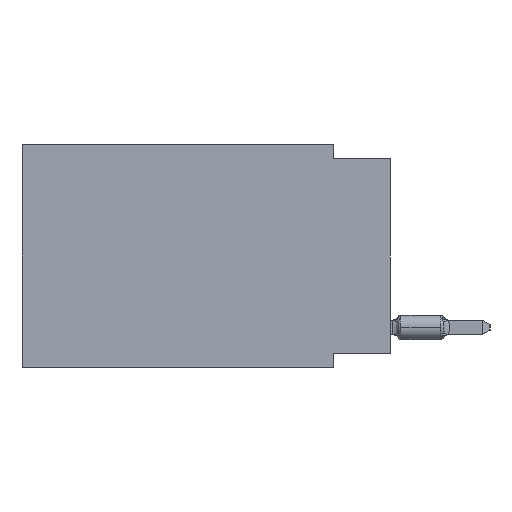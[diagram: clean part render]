
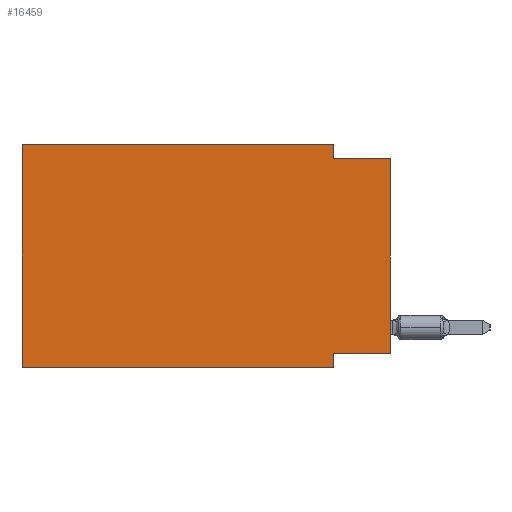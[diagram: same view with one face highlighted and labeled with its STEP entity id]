
A CAD part, left-side view. The second image highlights one B-rep face of the part: STEP entity #16459.
In plain terms, the highlighted planar face has unit normal (-1, 0, 0).
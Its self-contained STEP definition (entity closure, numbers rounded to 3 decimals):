
#486 = EDGE_CURVE ( 'NONE', #56220, #3566, #26985, .T. ) ;
#1985 = CARTESIAN_POINT ( 'NONE',  ( 0., 0., 0. ) ) ;
#2915 = ORIENTED_EDGE ( 'NONE', *, *, #71322, .F. ) ;
#3430 = PLANE ( 'NONE',  #68367 ) ;
#3566 = VERTEX_POINT ( 'NONE', #26659 ) ;
#4376 = VECTOR ( 'NONE', #16725, 1000. ) ;
#4615 = VERTEX_POINT ( 'NONE', #43589 ) ;
#5966 = CARTESIAN_POINT ( 'NONE',  ( 0., 0., -0.635 ) ) ;
#5991 = VERTEX_POINT ( 'NONE', #57848 ) ;
#6967 = VECTOR ( 'NONE', #25536, 1000. ) ;
#7829 = LINE ( 'NONE', #36813, #31061 ) ;
#8738 = CARTESIAN_POINT ( 'NONE',  ( 0., 2.54, -0.635 ) ) ;
#9152 = LINE ( 'NONE', #67476, #35748 ) ;
#10105 = VECTOR ( 'NONE', #44324, 1000. ) ;
#14427 = CARTESIAN_POINT ( 'NONE',  ( 0., 2.54, -9.906 ) ) ;
#15564 = EDGE_CURVE ( 'NONE', #56220, #51769, #19150, .T. ) ;
#15979 = LINE ( 'NONE', #45315, #4376 ) ;
#16459 = ADVANCED_FACE ( 'NONE', ( #54260 ), #3430, .F. ) ;
#16725 = DIRECTION ( 'NONE',  ( 0., -1., 0. ) ) ;
#19124 = DIRECTION ( 'NONE',  ( 0., 0., -1. ) ) ;
#19150 = LINE ( 'NONE', #37577, #6967 ) ;
#19627 = EDGE_CURVE ( 'NONE', #5991, #39199, #70482, .T. ) ;
#21343 = CARTESIAN_POINT ( 'NONE',  ( 0., 0., -0.635 ) ) ;
#25536 = DIRECTION ( 'NONE',  ( 0., -1., 0. ) ) ;
#25578 = VECTOR ( 'NONE', #36987, 1000. ) ;
#26659 = CARTESIAN_POINT ( 'NONE',  ( 0., 16.383, 0. ) ) ;
#26985 = LINE ( 'NONE', #48861, #59448 ) ;
#31061 = VECTOR ( 'NONE', #19124, 1000. ) ;
#31166 = VECTOR ( 'NONE', #58721, 1000. ) ;
#31665 = DIRECTION ( 'NONE',  ( 1., 0., 0. ) ) ;
#32376 = EDGE_LOOP ( 'NONE', ( #68929, #44259, #65101, #42489, #46317, #44425, #48082, #2915 ) ) ;
#34669 = LINE ( 'NONE', #35780, #31166 ) ;
#35748 = VECTOR ( 'NONE', #38874, 1000. ) ;
#35780 = CARTESIAN_POINT ( 'NONE',  ( 0., 2.54, -9.906 ) ) ;
#36478 = EDGE_CURVE ( 'NONE', #4615, #60180, #7829, .T. ) ;
#36813 = CARTESIAN_POINT ( 'NONE',  ( 0., 2.54, 0. ) ) ;
#36987 = DIRECTION ( 'NONE',  ( 0., 0., 1. ) ) ;
#37563 = DIRECTION ( 'NONE',  ( 0., 0., 1. ) ) ;
#37577 = CARTESIAN_POINT ( 'NONE',  ( 0., 16.383, -9.906 ) ) ;
#38801 = EDGE_CURVE ( 'NONE', #50393, #51769, #34669, .T. ) ;
#38874 = DIRECTION ( 'NONE',  ( 0., 1., 0. ) ) ;
#39199 = VERTEX_POINT ( 'NONE', #5966 ) ;
#41608 = CARTESIAN_POINT ( 'NONE',  ( 0., 16.383, -9.906 ) ) ;
#42489 = ORIENTED_EDGE ( 'NONE', *, *, #46061, .F. ) ;
#43589 = CARTESIAN_POINT ( 'NONE',  ( 0., 2.54, 0. ) ) ;
#44259 = ORIENTED_EDGE ( 'NONE', *, *, #67642, .F. ) ;
#44324 = DIRECTION ( 'NONE',  ( 0., -1., 0. ) ) ;
#44425 = ORIENTED_EDGE ( 'NONE', *, *, #15564, .T. ) ;
#45315 = CARTESIAN_POINT ( 'NONE',  ( 0., 16.383, 0. ) ) ;
#45432 = LINE ( 'NONE', #21343, #10105 ) ;
#46061 = EDGE_CURVE ( 'NONE', #3566, #4615, #15979, .T. ) ;
#46317 = ORIENTED_EDGE ( 'NONE', *, *, #486, .F. ) ;
#47083 = CARTESIAN_POINT ( 'NONE',  ( 0., 2.54, -9.271 ) ) ;
#48082 = ORIENTED_EDGE ( 'NONE', *, *, #38801, .F. ) ;
#48861 = CARTESIAN_POINT ( 'NONE',  ( 0., 16.383, 0. ) ) ;
#50393 = VERTEX_POINT ( 'NONE', #47083 ) ;
#51769 = VERTEX_POINT ( 'NONE', #14427 ) ;
#54260 = FACE_OUTER_BOUND ( 'NONE', #32376, .T. ) ;
#54984 = DIRECTION ( 'NONE',  ( 0., 0., -1. ) ) ;
#56220 = VERTEX_POINT ( 'NONE', #41608 ) ;
#57848 = CARTESIAN_POINT ( 'NONE',  ( 0., 0., -9.271 ) ) ;
#58721 = DIRECTION ( 'NONE',  ( 0., 0., -1. ) ) ;
#59448 = VECTOR ( 'NONE', #37563, 1000. ) ;
#60180 = VERTEX_POINT ( 'NONE', #8738 ) ;
#60616 = CARTESIAN_POINT ( 'NONE',  ( 0., 16.383, 0. ) ) ;
#65101 = ORIENTED_EDGE ( 'NONE', *, *, #36478, .F. ) ;
#67476 = CARTESIAN_POINT ( 'NONE',  ( 0., 0., -9.271 ) ) ;
#67642 = EDGE_CURVE ( 'NONE', #60180, #39199, #45432, .T. ) ;
#68367 = AXIS2_PLACEMENT_3D ( 'NONE', #60616, #31665, #54984 ) ;
#68929 = ORIENTED_EDGE ( 'NONE', *, *, #19627, .T. ) ;
#70482 = LINE ( 'NONE', #1985, #25578 ) ;
#71322 = EDGE_CURVE ( 'NONE', #5991, #50393, #9152, .T. ) ;
